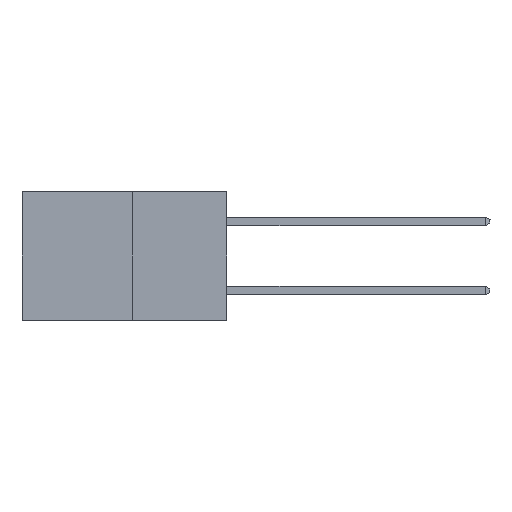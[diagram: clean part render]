
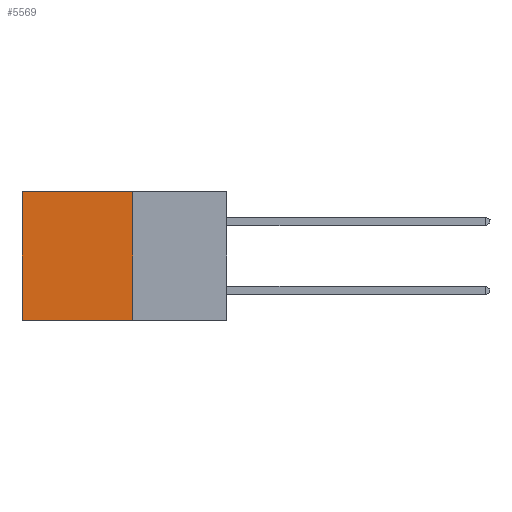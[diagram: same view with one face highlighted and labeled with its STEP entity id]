
A CAD part, left-side view. The second image highlights one B-rep face of the part: STEP entity #5569.
In plain terms, the highlighted planar face has unit normal (-1, 0, 0).
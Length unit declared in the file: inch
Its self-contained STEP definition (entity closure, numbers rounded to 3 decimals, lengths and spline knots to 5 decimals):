
#63 = VERTEX_POINT ( 'NONE', #3439 ) ;
#485 = CARTESIAN_POINT ( 'NONE',  ( 0.277, 0.27, -0.37 ) ) ;
#927 = EDGE_CURVE ( 'NONE', #63, #6934, #3334, .T. ) ;
#969 = VECTOR ( 'NONE', #8306, 39.37008 ) ;
#1294 = VECTOR ( 'NONE', #5685, 39.37008 ) ;
#1314 = DIRECTION ( 'NONE',  ( 0., 0., -1. ) ) ;
#1520 = CARTESIAN_POINT ( 'NONE',  ( 0.277, 0.59, -0.37 ) ) ;
#2162 = LINE ( 'NONE', #3109, #4501 ) ;
#2314 = DIRECTION ( 'NONE',  ( 1., 0., 0. ) ) ;
#3109 = CARTESIAN_POINT ( 'NONE',  ( 0.277, 0.27, -0.37 ) ) ;
#3110 = CARTESIAN_POINT ( 'NONE',  ( 0.277, 0.59, -0.37 ) ) ;
#3285 = ORIENTED_EDGE ( 'NONE', *, *, #11274, .T. ) ;
#3334 = LINE ( 'NONE', #9020, #969 ) ;
#3439 = CARTESIAN_POINT ( 'NONE',  ( 0.277, 0.27, -0.37 ) ) ;
#3928 = EDGE_LOOP ( 'NONE', ( #3285, #5597, #8000, #10361 ) ) ;
#4295 = EDGE_CURVE ( 'NONE', #8764, #63, #2162, .T. ) ;
#4501 = VECTOR ( 'NONE', #1314, 39.37008 ) ;
#4578 = DIRECTION ( 'NONE',  ( 0., 1., 0. ) ) ;
#5569 = ADVANCED_FACE ( 'NONE', ( #6319 ), #9366, .F. ) ;
#5597 = ORIENTED_EDGE ( 'NONE', *, *, #927, .F. ) ;
#5656 = CARTESIAN_POINT ( 'NONE',  ( 0.277, 0.27, 0. ) ) ;
#5685 = DIRECTION ( 'NONE',  ( 0., 0., -1. ) ) ;
#5987 = LINE ( 'NONE', #3110, #1294 ) ;
#6319 = FACE_OUTER_BOUND ( 'NONE', #3928, .T. ) ;
#6785 = VERTEX_POINT ( 'NONE', #10799 ) ;
#6842 = VECTOR ( 'NONE', #4578, 39.37008 ) ;
#6934 = VERTEX_POINT ( 'NONE', #1520 ) ;
#7115 = LINE ( 'NONE', #9015, #6842 ) ;
#8000 = ORIENTED_EDGE ( 'NONE', *, *, #4295, .F. ) ;
#8306 = DIRECTION ( 'NONE',  ( 0., 1., 0. ) ) ;
#8508 = DIRECTION ( 'NONE',  ( 0., 0., -1. ) ) ;
#8578 = EDGE_CURVE ( 'NONE', #8764, #6785, #7115, .T. ) ;
#8764 = VERTEX_POINT ( 'NONE', #5656 ) ;
#9015 = CARTESIAN_POINT ( 'NONE',  ( 0.277, 0.27, 0. ) ) ;
#9020 = CARTESIAN_POINT ( 'NONE',  ( 0.277, 0.27, -0.37 ) ) ;
#9366 = PLANE ( 'NONE',  #10929 ) ;
#10361 = ORIENTED_EDGE ( 'NONE', *, *, #8578, .T. ) ;
#10799 = CARTESIAN_POINT ( 'NONE',  ( 0.277, 0.59, 0. ) ) ;
#10929 = AXIS2_PLACEMENT_3D ( 'NONE', #485, #2314, #8508 ) ;
#11274 = EDGE_CURVE ( 'NONE', #6785, #6934, #5987, .T. ) ;
